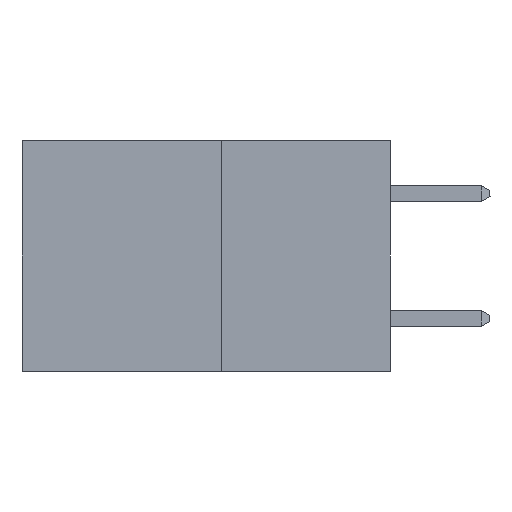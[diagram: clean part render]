
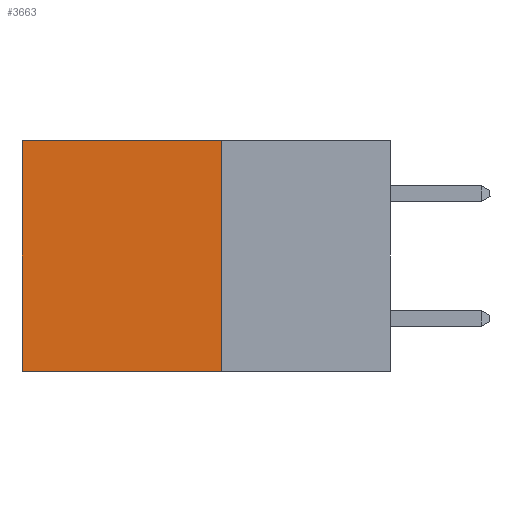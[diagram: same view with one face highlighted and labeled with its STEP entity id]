
A CAD part, left-side view. The second image highlights one B-rep face of the part: STEP entity #3663.
In plain terms, the highlighted planar face has unit normal (-1, 0, 0).
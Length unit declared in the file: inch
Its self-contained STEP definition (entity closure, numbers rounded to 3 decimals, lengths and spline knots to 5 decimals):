
#247 = VECTOR ( 'NONE', #13780, 39.37008 ) ;
#1774 = EDGE_CURVE ( 'NONE', #14882, #6754, #8982, .T. ) ;
#1942 = CARTESIAN_POINT ( 'NONE',  ( 0.277, 0.59, 0. ) ) ;
#2732 = VECTOR ( 'NONE', #4764, 39.37008 ) ;
#2767 = EDGE_CURVE ( 'NONE', #9608, #14882, #3054, .T. ) ;
#3054 = LINE ( 'NONE', #5536, #8952 ) ;
#3663 = ADVANCED_FACE ( 'NONE', ( #13353 ), #3934, .F. ) ;
#3934 = PLANE ( 'NONE',  #4827 ) ;
#4412 = CARTESIAN_POINT ( 'NONE',  ( 0.277, 0.27, -0.37 ) ) ;
#4764 = DIRECTION ( 'NONE',  ( 0., 0., -1. ) ) ;
#4827 = AXIS2_PLACEMENT_3D ( 'NONE', #13315, #6315, #14456 ) ;
#5236 = DIRECTION ( 'NONE',  ( 0., 1., 0. ) ) ;
#5536 = CARTESIAN_POINT ( 'NONE',  ( 0.277, 0.27, 0. ) ) ;
#5586 = CARTESIAN_POINT ( 'NONE',  ( 0.277, 0.27, -0.37 ) ) ;
#6315 = DIRECTION ( 'NONE',  ( 1., 0., 0. ) ) ;
#6754 = VERTEX_POINT ( 'NONE', #12869 ) ;
#7185 = ORIENTED_EDGE ( 'NONE', *, *, #1774, .T. ) ;
#7547 = ORIENTED_EDGE ( 'NONE', *, *, #12672, .F. ) ;
#8481 = VERTEX_POINT ( 'NONE', #14564 ) ;
#8952 = VECTOR ( 'NONE', #5236, 39.37008 ) ;
#8982 = LINE ( 'NONE', #11729, #2732 ) ;
#9394 = LINE ( 'NONE', #4412, #14794 ) ;
#9608 = VERTEX_POINT ( 'NONE', #14402 ) ;
#10319 = EDGE_LOOP ( 'NONE', ( #7185, #13349, #7547, #10617 ) ) ;
#10617 = ORIENTED_EDGE ( 'NONE', *, *, #2767, .T. ) ;
#11467 = DIRECTION ( 'NONE',  ( 0., 1., 0. ) ) ;
#11729 = CARTESIAN_POINT ( 'NONE',  ( 0.277, 0.59, -0.37 ) ) ;
#12135 = LINE ( 'NONE', #5586, #247 ) ;
#12672 = EDGE_CURVE ( 'NONE', #9608, #8481, #12135, .T. ) ;
#12691 = EDGE_CURVE ( 'NONE', #8481, #6754, #9394, .T. ) ;
#12869 = CARTESIAN_POINT ( 'NONE',  ( 0.277, 0.59, -0.37 ) ) ;
#13315 = CARTESIAN_POINT ( 'NONE',  ( 0.277, 0.27, -0.37 ) ) ;
#13349 = ORIENTED_EDGE ( 'NONE', *, *, #12691, .F. ) ;
#13353 = FACE_OUTER_BOUND ( 'NONE', #10319, .T. ) ;
#13780 = DIRECTION ( 'NONE',  ( 0., 0., -1. ) ) ;
#14402 = CARTESIAN_POINT ( 'NONE',  ( 0.277, 0.27, 0. ) ) ;
#14456 = DIRECTION ( 'NONE',  ( 0., 0., -1. ) ) ;
#14564 = CARTESIAN_POINT ( 'NONE',  ( 0.277, 0.27, -0.37 ) ) ;
#14794 = VECTOR ( 'NONE', #11467, 39.37008 ) ;
#14882 = VERTEX_POINT ( 'NONE', #1942 ) ;
